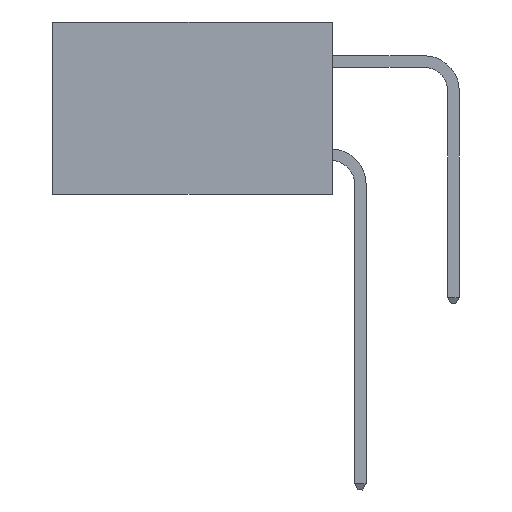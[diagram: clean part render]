
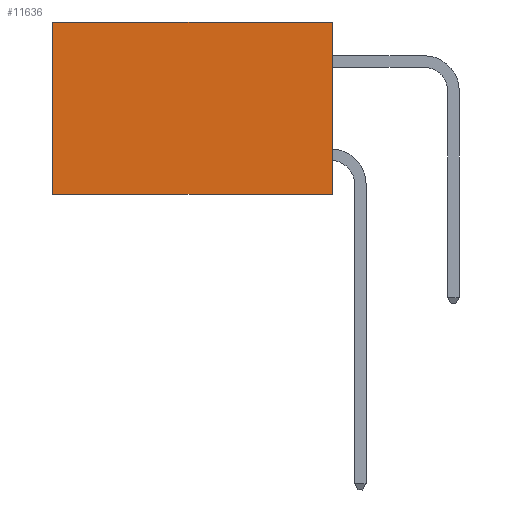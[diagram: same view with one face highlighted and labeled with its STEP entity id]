
A CAD part, left-side view. The second image highlights one B-rep face of the part: STEP entity #11636.
In plain terms, the highlighted planar face has unit normal (-1, 0, 0).
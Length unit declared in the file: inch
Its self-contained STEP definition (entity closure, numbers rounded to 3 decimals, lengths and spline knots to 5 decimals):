
#799 = ORIENTED_EDGE ( 'NONE', *, *, #4618, .F. ) ;
#1657 = ORIENTED_EDGE ( 'NONE', *, *, #4783, .F. ) ;
#2029 = VERTEX_POINT ( 'NONE', #3145 ) ;
#2068 = FACE_OUTER_BOUND ( 'NONE', #9855, .T. ) ;
#2869 = EDGE_CURVE ( 'NONE', #2029, #11291, #4522, .T. ) ;
#3145 = CARTESIAN_POINT ( 'NONE',  ( 0.298, 0., 0. ) ) ;
#4140 = CARTESIAN_POINT ( 'NONE',  ( 0.298, 0., -0.37 ) ) ;
#4502 = VERTEX_POINT ( 'NONE', #7868 ) ;
#4522 = LINE ( 'NONE', #6964, #10304 ) ;
#4618 = EDGE_CURVE ( 'NONE', #2029, #10276, #9790, .T. ) ;
#4783 = EDGE_CURVE ( 'NONE', #10276, #4502, #12589, .T. ) ;
#4832 = DIRECTION ( 'NONE',  ( 0., 0., -1. ) ) ;
#4842 = PLANE ( 'NONE',  #7173 ) ;
#5206 = CARTESIAN_POINT ( 'NONE',  ( 0.298, 0., 0. ) ) ;
#6020 = DIRECTION ( 'NONE',  ( 0., 0., -1. ) ) ;
#6418 = VECTOR ( 'NONE', #11209, 39.37008 ) ;
#6964 = CARTESIAN_POINT ( 'NONE',  ( 0.298, 0., 0. ) ) ;
#7173 = AXIS2_PLACEMENT_3D ( 'NONE', #13831, #12801, #6020 ) ;
#7538 = DIRECTION ( 'NONE',  ( 0., 1., 0. ) ) ;
#7868 = CARTESIAN_POINT ( 'NONE',  ( 0.298, 0.6, -0.37 ) ) ;
#8516 = ORIENTED_EDGE ( 'NONE', *, *, #2869, .T. ) ;
#8885 = VECTOR ( 'NONE', #4832, 39.37008 ) ;
#9051 = CARTESIAN_POINT ( 'NONE',  ( 0.298, 0., -0.37 ) ) ;
#9423 = DIRECTION ( 'NONE',  ( 0., 1., 0. ) ) ;
#9790 = LINE ( 'NONE', #5206, #6418 ) ;
#9855 = EDGE_LOOP ( 'NONE', ( #14099, #1657, #799, #8516 ) ) ;
#9969 = VECTOR ( 'NONE', #9423, 39.37008 ) ;
#10268 = CARTESIAN_POINT ( 'NONE',  ( 0.298, 0.6, 0. ) ) ;
#10276 = VERTEX_POINT ( 'NONE', #4140 ) ;
#10304 = VECTOR ( 'NONE', #7538, 39.37008 ) ;
#10562 = EDGE_CURVE ( 'NONE', #11291, #4502, #11574, .T. ) ;
#11209 = DIRECTION ( 'NONE',  ( 0., 0., -1. ) ) ;
#11291 = VERTEX_POINT ( 'NONE', #10268 ) ;
#11574 = LINE ( 'NONE', #11700, #8885 ) ;
#11636 = ADVANCED_FACE ( 'NONE', ( #2068 ), #4842, .F. ) ;
#11700 = CARTESIAN_POINT ( 'NONE',  ( 0.298, 0.6, 0. ) ) ;
#12589 = LINE ( 'NONE', #9051, #9969 ) ;
#12801 = DIRECTION ( 'NONE',  ( 1., 0., 0. ) ) ;
#13831 = CARTESIAN_POINT ( 'NONE',  ( 0.298, 0., 0. ) ) ;
#14099 = ORIENTED_EDGE ( 'NONE', *, *, #10562, .T. ) ;
